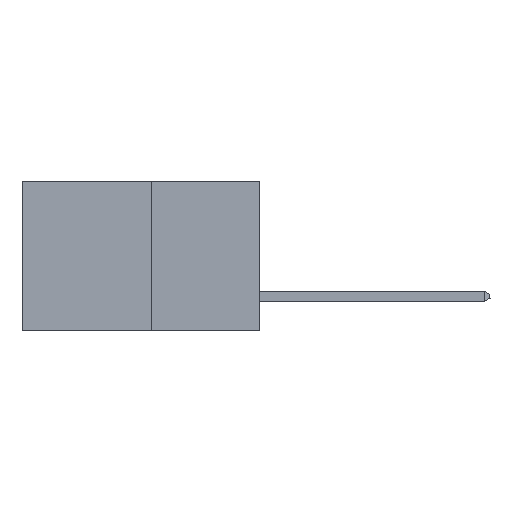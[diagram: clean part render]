
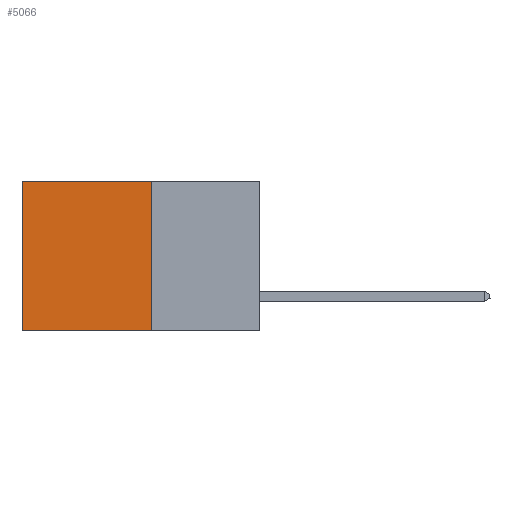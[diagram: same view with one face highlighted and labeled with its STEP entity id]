
A CAD part, left-side view. The second image highlights one B-rep face of the part: STEP entity #5066.
In plain terms, the highlighted planar face has unit normal (-1, 0, 0).
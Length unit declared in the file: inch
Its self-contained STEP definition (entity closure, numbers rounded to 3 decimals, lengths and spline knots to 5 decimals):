
#130 = LINE ( 'NONE', #9388, #12973 ) ;
#1569 = CARTESIAN_POINT ( 'NONE',  ( 0.277, 0.27, -0.37 ) ) ;
#1583 = LINE ( 'NONE', #5841, #14548 ) ;
#3225 = VECTOR ( 'NONE', #9477, 39.37008 ) ;
#3318 = CARTESIAN_POINT ( 'NONE',  ( 0.277, 0.27, -0.37 ) ) ;
#3366 = VECTOR ( 'NONE', #10036, 39.37008 ) ;
#3443 = FACE_OUTER_BOUND ( 'NONE', #11884, .T. ) ;
#3615 = LINE ( 'NONE', #3318, #3225 ) ;
#3770 = CARTESIAN_POINT ( 'NONE',  ( 0.277, 0.59, -0.37 ) ) ;
#5066 = ADVANCED_FACE ( 'NONE', ( #3443 ), #15048, .F. ) ;
#5651 = DIRECTION ( 'NONE',  ( 0., 0., -1. ) ) ;
#5652 = VERTEX_POINT ( 'NONE', #15238 ) ;
#5841 = CARTESIAN_POINT ( 'NONE',  ( 0.277, 0.27, 0. ) ) ;
#6041 = ORIENTED_EDGE ( 'NONE', *, *, #12536, .F. ) ;
#6091 = ORIENTED_EDGE ( 'NONE', *, *, #15294, .F. ) ;
#6105 = ORIENTED_EDGE ( 'NONE', *, *, #11689, .T. ) ;
#6370 = CARTESIAN_POINT ( 'NONE',  ( 0.277, 0.27, -0.37 ) ) ;
#7603 = VERTEX_POINT ( 'NONE', #13542 ) ;
#8013 = CARTESIAN_POINT ( 'NONE',  ( 0.277, 0.59, 0. ) ) ;
#8043 = VERTEX_POINT ( 'NONE', #8013 ) ;
#8236 = DIRECTION ( 'NONE',  ( 1., 0., 0. ) ) ;
#8865 = EDGE_CURVE ( 'NONE', #7603, #8043, #1583, .T. ) ;
#9388 = CARTESIAN_POINT ( 'NONE',  ( 0.277, 0.59, -0.37 ) ) ;
#9477 = DIRECTION ( 'NONE',  ( 0., 0., -1. ) ) ;
#9624 = AXIS2_PLACEMENT_3D ( 'NONE', #1569, #8236, #13313 ) ;
#10036 = DIRECTION ( 'NONE',  ( 0., 1., 0. ) ) ;
#10524 = ORIENTED_EDGE ( 'NONE', *, *, #8865, .T. ) ;
#11265 = VERTEX_POINT ( 'NONE', #3770 ) ;
#11689 = EDGE_CURVE ( 'NONE', #8043, #11265, #130, .T. ) ;
#11884 = EDGE_LOOP ( 'NONE', ( #6105, #6091, #6041, #10524 ) ) ;
#12536 = EDGE_CURVE ( 'NONE', #7603, #5652, #3615, .T. ) ;
#12973 = VECTOR ( 'NONE', #5651, 39.37008 ) ;
#13313 = DIRECTION ( 'NONE',  ( 0., 0., -1. ) ) ;
#13542 = CARTESIAN_POINT ( 'NONE',  ( 0.277, 0.27, 0. ) ) ;
#14520 = DIRECTION ( 'NONE',  ( 0., 1., 0. ) ) ;
#14548 = VECTOR ( 'NONE', #14520, 39.37008 ) ;
#15048 = PLANE ( 'NONE',  #9624 ) ;
#15238 = CARTESIAN_POINT ( 'NONE',  ( 0.277, 0.27, -0.37 ) ) ;
#15294 = EDGE_CURVE ( 'NONE', #5652, #11265, #15726, .T. ) ;
#15726 = LINE ( 'NONE', #6370, #3366 ) ;
